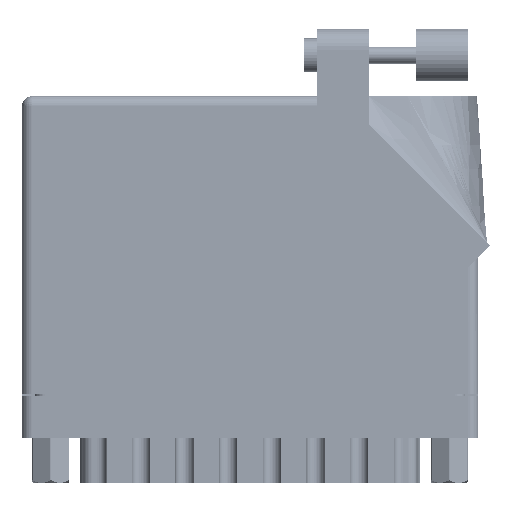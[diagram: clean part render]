
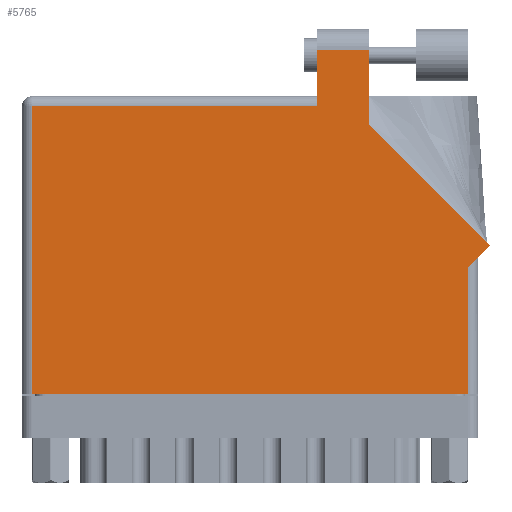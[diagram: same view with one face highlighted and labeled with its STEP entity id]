
A CAD part, front view. The second image highlights one B-rep face of the part: STEP entity #5765.
In plain terms, the highlighted face is planar.
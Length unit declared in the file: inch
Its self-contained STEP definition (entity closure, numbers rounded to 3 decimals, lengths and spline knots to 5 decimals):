
#1616 = ORIENTED_EDGE ( 'NONE', *, *, #85529, .T. ) ;
#2574 = CARTESIAN_POINT ( 'NONE',  ( 0., 1.713, 0. ) ) ;
#3900 = CARTESIAN_POINT ( 'NONE',  ( 1.758, 1.713, 0. ) ) ;
#5765 = ADVANCED_FACE ( 'NONE', ( #29178 ), #84562, .F. ) ;
#8200 = DIRECTION ( 'NONE',  ( -0.707, 0.707, 0. ) ) ;
#8865 = LINE ( 'NONE', #2574, #77501 ) ;
#9394 = VERTEX_POINT ( 'NONE', #61502 ) ;
#10649 = CARTESIAN_POINT ( 'NONE',  ( 2.656, 0.815, 0. ) ) ;
#11382 = VECTOR ( 'NONE', #22042, 39.37008 ) ;
#12038 = VECTOR ( 'NONE', #59439, 39.37008 ) ;
#12232 = DIRECTION ( 'NONE',  ( -1., 0., 0. ) ) ;
#12956 = CARTESIAN_POINT ( 'NONE',  ( 2.065, 1.60942, 0. ) ) ;
#13692 = EDGE_CURVE ( 'NONE', #17045, #70506, #60076, .T. ) ;
#14148 = DIRECTION ( 'NONE',  ( 0., 1., 0. ) ) ;
#14639 = EDGE_CURVE ( 'NONE', #70506, #32841, #84803, .T. ) ;
#16182 = LINE ( 'NONE', #40366, #35963 ) ;
#16331 = VECTOR ( 'NONE', #19784, 39.37008 ) ;
#16981 = EDGE_CURVE ( 'NONE', #32841, #9394, #70014, .T. ) ;
#17045 = VERTEX_POINT ( 'NONE', #58252 ) ;
#17788 = ORIENTED_EDGE ( 'NONE', *, *, #16981, .T. ) ;
#18785 = CARTESIAN_POINT ( 'NONE',  ( 2.656, 0.753, 0. ) ) ;
#19784 = DIRECTION ( 'NONE',  ( 0.707, 0.707, 0. ) ) ;
#21042 = ORIENTED_EDGE ( 'NONE', *, *, #33983, .T. ) ;
#21514 = DIRECTION ( 'NONE',  ( -1., 0., 0. ) ) ;
#21722 = DIRECTION ( 'NONE',  ( 0., -1., 0. ) ) ;
#22042 = DIRECTION ( 'NONE',  ( 1., 0., 0. ) ) ;
#26433 = AXIS2_PLACEMENT_3D ( 'NONE', #44809, #52041, #12232 ) ;
#29178 = FACE_OUTER_BOUND ( 'NONE', #52616, .T. ) ;
#32841 = VERTEX_POINT ( 'NONE', #66663 ) ;
#33983 = EDGE_CURVE ( 'NONE', #46440, #47378, #41243, .T. ) ;
#34558 = EDGE_CURVE ( 'NONE', #79381, #46440, #8865, .T. ) ;
#34811 = LINE ( 'NONE', #10649, #70113 ) ;
#35963 = VECTOR ( 'NONE', #73217, 39.37008 ) ;
#38624 = EDGE_CURVE ( 'NONE', #47378, #66244, #67524, .T. ) ;
#38852 = VERTEX_POINT ( 'NONE', #18785 ) ;
#39039 = ORIENTED_EDGE ( 'NONE', *, *, #14639, .T. ) ;
#40321 = CARTESIAN_POINT ( 'NONE',  ( 0.062, 0., 0. ) ) ;
#40366 = CARTESIAN_POINT ( 'NONE',  ( 1.758, 1.775, 0. ) ) ;
#41243 = LINE ( 'NONE', #40321, #48605 ) ;
#42417 = VECTOR ( 'NONE', #8200, 39.37008 ) ;
#43432 = CARTESIAN_POINT ( 'NONE',  ( 2.656, 0., 0. ) ) ;
#44809 = CARTESIAN_POINT ( 'NONE',  ( 0., 1.775, 0. ) ) ;
#45113 = VECTOR ( 'NONE', #70764, 39.37008 ) ;
#46440 = VERTEX_POINT ( 'NONE', #76275 ) ;
#46764 = ORIENTED_EDGE ( 'NONE', *, *, #13692, .T. ) ;
#46805 = CARTESIAN_POINT ( 'NONE',  ( 2.718, 0.815, 0. ) ) ;
#47378 = VERTEX_POINT ( 'NONE', #76280 ) ;
#48605 = VECTOR ( 'NONE', #21722, 39.37008 ) ;
#48752 = ORIENTED_EDGE ( 'NONE', *, *, #69408, .T. ) ;
#50676 = LINE ( 'NONE', #46805, #16331 ) ;
#52041 = DIRECTION ( 'NONE',  ( 0., 0., -1. ) ) ;
#52616 = EDGE_LOOP ( 'NONE', ( #39039, #17788, #48752, #70019, #21042, #76843, #56180, #1616, #46764 ) ) ;
#55162 = CARTESIAN_POINT ( 'NONE',  ( 0., 0., 0. ) ) ;
#56180 = ORIENTED_EDGE ( 'NONE', *, *, #69917, .T. ) ;
#57117 = CARTESIAN_POINT ( 'NONE',  ( 1.758, 2.05, 0. ) ) ;
#58252 = CARTESIAN_POINT ( 'NONE',  ( 2.78871, 0.88571, 0. ) ) ;
#59439 = DIRECTION ( 'NONE',  ( 0., 1., 0. ) ) ;
#60076 = LINE ( 'NONE', #81119, #42417 ) ;
#61502 = CARTESIAN_POINT ( 'NONE',  ( 1.758, 2.05, 0. ) ) ;
#66244 = VERTEX_POINT ( 'NONE', #43432 ) ;
#66663 = CARTESIAN_POINT ( 'NONE',  ( 2.065, 2.05, 0. ) ) ;
#67524 = LINE ( 'NONE', #55162, #11382 ) ;
#69408 = EDGE_CURVE ( 'NONE', #9394, #79381, #16182, .T. ) ;
#69917 = EDGE_CURVE ( 'NONE', #66244, #38852, #34811, .T. ) ;
#70014 = LINE ( 'NONE', #57117, #45113 ) ;
#70019 = ORIENTED_EDGE ( 'NONE', *, *, #34558, .T. ) ;
#70113 = VECTOR ( 'NONE', #14148, 39.37008 ) ;
#70506 = VERTEX_POINT ( 'NONE', #86077 ) ;
#70764 = DIRECTION ( 'NONE',  ( -1., 0., 0. ) ) ;
#73217 = DIRECTION ( 'NONE',  ( 0., -1., 0. ) ) ;
#76275 = CARTESIAN_POINT ( 'NONE',  ( 0.062, 1.713, 0. ) ) ;
#76280 = CARTESIAN_POINT ( 'NONE',  ( 0.062, 0., 0. ) ) ;
#76843 = ORIENTED_EDGE ( 'NONE', *, *, #38624, .T. ) ;
#77501 = VECTOR ( 'NONE', #21514, 39.37008 ) ;
#79381 = VERTEX_POINT ( 'NONE', #3900 ) ;
#81119 = CARTESIAN_POINT ( 'NONE',  ( 2.78871, 0.88571, 0. ) ) ;
#84562 = PLANE ( 'NONE',  #26433 ) ;
#84803 = LINE ( 'NONE', #12956, #12038 ) ;
#85529 = EDGE_CURVE ( 'NONE', #38852, #17045, #50676, .T. ) ;
#86077 = CARTESIAN_POINT ( 'NONE',  ( 2.065, 1.60942, 0. ) ) ;
